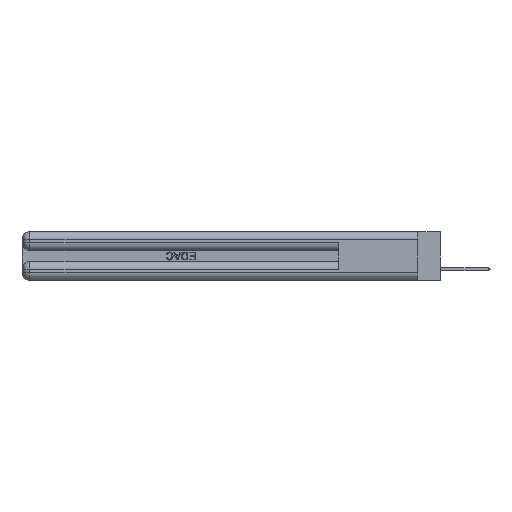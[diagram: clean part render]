
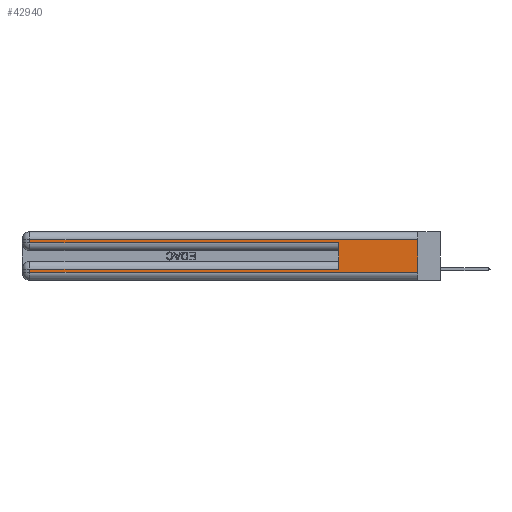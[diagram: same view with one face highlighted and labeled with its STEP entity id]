
A CAD part, left-side view. The second image highlights one B-rep face of the part: STEP entity #42940.
In plain terms, the highlighted planar face has unit normal (-1, 0, 0).
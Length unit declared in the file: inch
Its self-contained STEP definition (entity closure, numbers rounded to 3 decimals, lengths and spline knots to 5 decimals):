
#228 = CARTESIAN_POINT ( 'NONE',  ( 0., 0., 0.31 ) ) ;
#307 = EDGE_CURVE ( 'NONE', #29304, #39396, #37578, .T. ) ;
#1716 = VECTOR ( 'NONE', #37641, 39.37008 ) ;
#2414 = LINE ( 'NONE', #13064, #40985 ) ;
#2488 = LINE ( 'NONE', #17981, #41053 ) ;
#2681 = VECTOR ( 'NONE', #36834, 39.37008 ) ;
#2773 = DIRECTION ( 'NONE',  ( 0., 0., -1. ) ) ;
#2833 = CARTESIAN_POINT ( 'NONE',  ( 0., 2.94, 0.085 ) ) ;
#3088 = PLANE ( 'NONE',  #20338 ) ;
#3671 = EDGE_CURVE ( 'NONE', #20717, #37993, #2414, .T. ) ;
#3816 = LINE ( 'NONE', #22666, #30582 ) ;
#4852 = CARTESIAN_POINT ( 'NONE',  ( 0., 2.94, 0.06 ) ) ;
#4967 = CARTESIAN_POINT ( 'NONE',  ( 0., 0., 0.31 ) ) ;
#5217 = ORIENTED_EDGE ( 'NONE', *, *, #307, .T. ) ;
#6721 = VECTOR ( 'NONE', #28338, 39.37008 ) ;
#7003 = ORIENTED_EDGE ( 'NONE', *, *, #3671, .T. ) ;
#7546 = CARTESIAN_POINT ( 'NONE',  ( 0., 0., 0.37 ) ) ;
#8331 = EDGE_LOOP ( 'NONE', ( #25032, #5217, #20304, #31581, #42272, #39264, #7003, #28848 ) ) ;
#9865 = CARTESIAN_POINT ( 'NONE',  ( 0., 0., 0.285 ) ) ;
#9943 = DIRECTION ( 'NONE',  ( 0., 0., -1. ) ) ;
#11125 = CARTESIAN_POINT ( 'NONE',  ( 0., 0.6, 0.085 ) ) ;
#11298 = VECTOR ( 'NONE', #20436, 39.37008 ) ;
#11734 = CARTESIAN_POINT ( 'NONE',  ( 0., 2.94, 0.31 ) ) ;
#12477 = VECTOR ( 'NONE', #20786, 39.37008 ) ;
#13064 = CARTESIAN_POINT ( 'NONE',  ( 0., 2.94, 0.37 ) ) ;
#13691 = CARTESIAN_POINT ( 'NONE',  ( 0., 0., 0.085 ) ) ;
#15774 = LINE ( 'NONE', #7546, #6721 ) ;
#17981 = CARTESIAN_POINT ( 'NONE',  ( 0., 0., 0.06 ) ) ;
#19159 = DIRECTION ( 'NONE',  ( 0., 0., -1. ) ) ;
#19383 = EDGE_CURVE ( 'NONE', #39396, #34511, #3816, .T. ) ;
#20304 = ORIENTED_EDGE ( 'NONE', *, *, #19383, .T. ) ;
#20338 = AXIS2_PLACEMENT_3D ( 'NONE', #30465, #37501, #9943 ) ;
#20436 = DIRECTION ( 'NONE',  ( 0., 1., 0. ) ) ;
#20717 = VERTEX_POINT ( 'NONE', #2833 ) ;
#20786 = DIRECTION ( 'NONE',  ( 0., 0., 1. ) ) ;
#22457 = LINE ( 'NONE', #9865, #2681 ) ;
#22666 = CARTESIAN_POINT ( 'NONE',  ( 0., 2.94, 0.37 ) ) ;
#23186 = LINE ( 'NONE', #37852, #12477 ) ;
#24045 = VERTEX_POINT ( 'NONE', #11125 ) ;
#25032 = ORIENTED_EDGE ( 'NONE', *, *, #32866, .F. ) ;
#25386 = EDGE_CURVE ( 'NONE', #34511, #40193, #22457, .T. ) ;
#28338 = DIRECTION ( 'NONE',  ( 0., 0., -1. ) ) ;
#28848 = ORIENTED_EDGE ( 'NONE', *, *, #32117, .T. ) ;
#29021 = LINE ( 'NONE', #13691, #1716 ) ;
#29304 = VERTEX_POINT ( 'NONE', #4967 ) ;
#30208 = EDGE_CURVE ( 'NONE', #24045, #20717, #29021, .T. ) ;
#30465 = CARTESIAN_POINT ( 'NONE',  ( 0., 0., 0.37 ) ) ;
#30582 = VECTOR ( 'NONE', #2773, 39.37008 ) ;
#31581 = ORIENTED_EDGE ( 'NONE', *, *, #25386, .T. ) ;
#31917 = FACE_OUTER_BOUND ( 'NONE', #8331, .T. ) ;
#32027 = DIRECTION ( 'NONE',  ( 0., -1., 0. ) ) ;
#32117 = EDGE_CURVE ( 'NONE', #37993, #33737, #2488, .T. ) ;
#32866 = EDGE_CURVE ( 'NONE', #29304, #33737, #15774, .T. ) ;
#33081 = CARTESIAN_POINT ( 'NONE',  ( 0., 0.6, 0.285 ) ) ;
#33737 = VERTEX_POINT ( 'NONE', #40737 ) ;
#33954 = EDGE_CURVE ( 'NONE', #24045, #40193, #23186, .T. ) ;
#34511 = VERTEX_POINT ( 'NONE', #44144 ) ;
#36834 = DIRECTION ( 'NONE',  ( 0., -1., 0. ) ) ;
#37501 = DIRECTION ( 'NONE',  ( 1., 0., 0. ) ) ;
#37578 = LINE ( 'NONE', #228, #11298 ) ;
#37641 = DIRECTION ( 'NONE',  ( 0., 1., 0. ) ) ;
#37852 = CARTESIAN_POINT ( 'NONE',  ( 0., 0.6, 0.145 ) ) ;
#37993 = VERTEX_POINT ( 'NONE', #4852 ) ;
#39264 = ORIENTED_EDGE ( 'NONE', *, *, #30208, .T. ) ;
#39396 = VERTEX_POINT ( 'NONE', #11734 ) ;
#40193 = VERTEX_POINT ( 'NONE', #33081 ) ;
#40737 = CARTESIAN_POINT ( 'NONE',  ( 0., 0., 0.06 ) ) ;
#40985 = VECTOR ( 'NONE', #19159, 39.37008 ) ;
#41053 = VECTOR ( 'NONE', #32027, 39.37008 ) ;
#42272 = ORIENTED_EDGE ( 'NONE', *, *, #33954, .F. ) ;
#42940 = ADVANCED_FACE ( 'NONE', ( #31917 ), #3088, .F. ) ;
#44144 = CARTESIAN_POINT ( 'NONE',  ( 0., 2.94, 0.285 ) ) ;
